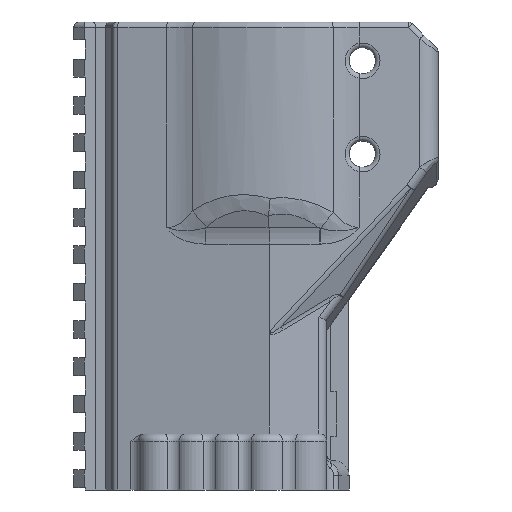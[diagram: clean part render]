
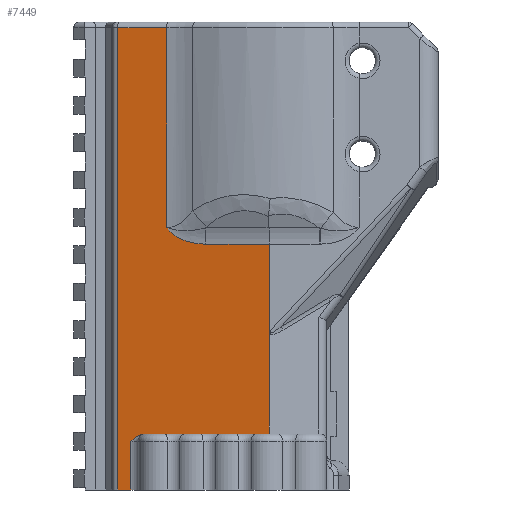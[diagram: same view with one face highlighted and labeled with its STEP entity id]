
A CAD part, left-side view. The second image highlights one B-rep face of the part: STEP entity #7449.
In plain terms, the highlighted planar face has unit normal (-0.979, 0.206, 0).
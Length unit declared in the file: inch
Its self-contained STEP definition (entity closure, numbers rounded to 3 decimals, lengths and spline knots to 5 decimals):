
#97=B_SPLINE_CURVE_WITH_KNOTS('',3,(#11676,#11677,#11678,#11679,#11680,
#11681,#11682,#11683,#11684,#11685),.UNSPECIFIED.,.F.,.F.,(4,2,2,2,4),(0.,
0.1281,0.2562,0.33578,0.41537),
 .UNSPECIFIED.);
#139=B_SPLINE_CURVE_WITH_KNOTS('',3,(#13659,#13660,#13661,#13662,#13663,
#13664,#13665,#13666,#13667,#13668,#13669,#13670),.UNSPECIFIED.,.F.,.F.,
(4,2,1,1,1,1,1,1,4),(-1.20029,-1.19791,-0.95833,
-0.83854,-0.71875,-0.59896,-0.47916,
-0.23958,0.),.UNSPECIFIED.);
#303=PLANE('',#8259);
#616=FACE_OUTER_BOUND('',#1063,.T.);
#1063=EDGE_LOOP('',(#6061,#6062,#6063,#6064,#6065,#6066,#6067,#6068,#6069,
#6070,#6071));
#1374=LINE('',#10904,#1981);
#1447=LINE('',#11693,#2054);
#1635=LINE('',#12760,#2242);
#1694=LINE('',#13674,#2301);
#1699=LINE('',#13939,#2306);
#1700=LINE('',#13941,#2307);
#1701=LINE('',#13942,#2308);
#1702=LINE('',#13943,#2309);
#1703=LINE('',#13944,#2310);
#1981=VECTOR('',#8602,0.3937);
#2054=VECTOR('',#9099,0.3937);
#2242=VECTOR('',#9643,0.3937);
#2301=VECTOR('',#9954,0.3937);
#2306=VECTOR('',#10011,0.3937);
#2307=VECTOR('',#10012,0.3937);
#2308=VECTOR('',#10013,0.3937);
#2309=VECTOR('',#10014,0.3937);
#2310=VECTOR('',#10015,0.3937);
#2996=VERTEX_POINT('',#10901);
#2997=VERTEX_POINT('',#10903);
#3186=VERTEX_POINT('',#11674);
#3187=VERTEX_POINT('',#11675);
#3189=VERTEX_POINT('',#11691);
#3456=VERTEX_POINT('',#12757);
#3457=VERTEX_POINT('',#12759);
#3545=VERTEX_POINT('',#13643);
#3547=VERTEX_POINT('',#13646);
#3562=VERTEX_POINT('',#13938);
#3563=VERTEX_POINT('',#13940);
#3711=EDGE_CURVE('',#2997,#2996,#1374,.T.);
#3956=EDGE_CURVE('',#3186,#3187,#97,.F.);
#3961=EDGE_CURVE('',#3186,#3189,#1447,.T.);
#4296=EDGE_CURVE('',#3457,#3456,#1635,.T.);
#4451=EDGE_CURVE('',#3547,#3545,#139,.T.);
#4453=EDGE_CURVE('',#3545,#3456,#1694,.T.);
#4482=EDGE_CURVE('',#3562,#3547,#1699,.T.);
#4483=EDGE_CURVE('',#3563,#3562,#1700,.T.);
#4484=EDGE_CURVE('',#2997,#3563,#1701,.T.);
#4485=EDGE_CURVE('',#3187,#2996,#1702,.T.);
#4486=EDGE_CURVE('',#3189,#3457,#1703,.T.);
#6061=ORIENTED_EDGE('',*,*,#4451,.F.);
#6062=ORIENTED_EDGE('',*,*,#4482,.F.);
#6063=ORIENTED_EDGE('',*,*,#4483,.F.);
#6064=ORIENTED_EDGE('',*,*,#4484,.F.);
#6065=ORIENTED_EDGE('',*,*,#3711,.T.);
#6066=ORIENTED_EDGE('',*,*,#4485,.F.);
#6067=ORIENTED_EDGE('',*,*,#3956,.F.);
#6068=ORIENTED_EDGE('',*,*,#3961,.T.);
#6069=ORIENTED_EDGE('',*,*,#4486,.T.);
#6070=ORIENTED_EDGE('',*,*,#4296,.T.);
#6071=ORIENTED_EDGE('',*,*,#4453,.F.);
#7449=ADVANCED_FACE('',(#616),#303,.T.);
#8259=AXIS2_PLACEMENT_3D('',#13937,#10009,#10010);
#8602=DIRECTION('',(-0.206,-0.979,0.));
#9099=DIRECTION('',(-0.206,-0.979,0.));
#9643=DIRECTION('',(0.,0.,1.));
#9954=DIRECTION('',(-0.206,-0.979,0.));
#10009=DIRECTION('center_axis',(-0.979,0.206,0.));
#10010=DIRECTION('ref_axis',(-0.206,-0.979,0.));
#10011=DIRECTION('',(0.,0.,-1.));
#10012=DIRECTION('',(-0.206,-0.979,0.));
#10013=DIRECTION('',(0.,0.,1.));
#10014=DIRECTION('',(0.,0.,-1.));
#10015=DIRECTION('',(0.,0.,1.));
#10901=CARTESIAN_POINT('',(-0.76358,0.46364,5.49557));
#10903=CARTESIAN_POINT('',(-0.73495,0.59981,5.49557));
#10904=CARTESIAN_POINT('',(-0.88188,-0.09914,5.49557));
#11674=CARTESIAN_POINT('',(-0.79501,0.31412,6.08612));
#11675=CARTESIAN_POINT('',(-0.76358,0.46364,6.01112));
#11676=CARTESIAN_POINT('Ctrl Pts',(-0.76358,0.46364,
6.01112));
#11677=CARTESIAN_POINT('Ctrl Pts',(-0.76628,0.45077,
6.0216));
#11678=CARTESIAN_POINT('Ctrl Pts',(-0.76925,0.43663,
6.03315));
#11679=CARTESIAN_POINT('Ctrl Pts',(-0.77545,0.40717,
6.05432));
#11680=CARTESIAN_POINT('Ctrl Pts',(-0.77868,0.39178,
6.06384));
#11681=CARTESIAN_POINT('Ctrl Pts',(-0.78378,0.36752,
6.07516));
#11682=CARTESIAN_POINT('Ctrl Pts',(-0.78599,0.357,
6.07918));
#11683=CARTESIAN_POINT('Ctrl Pts',(-0.79053,0.33542,
6.08467));
#11684=CARTESIAN_POINT('Ctrl Pts',(-0.79286,0.32435,
6.08612));
#11685=CARTESIAN_POINT('Ctrl Pts',(-0.79501,0.31412,
6.08612));
#11691=CARTESIAN_POINT('',(-1.07106,-0.99901,6.08612));
#11693=CARTESIAN_POINT('',(-0.8733,-0.05833,6.08612));
#12757=CARTESIAN_POINT('',(-1.07106,-0.99901,8.08939));
#12759=CARTESIAN_POINT('',(-1.07106,-0.99901,7.14465));
#12760=CARTESIAN_POINT('',(-1.07106,-0.99901,-2.40157));
#13643=CARTESIAN_POINT('',(-0.93019,-0.3289,8.08939));
#13646=CARTESIAN_POINT('',(-0.84356,0.08314,8.26572));
#13659=CARTESIAN_POINT('Ctrl Pts',(-0.84356,0.08314,
8.26572));
#13660=CARTESIAN_POINT('Ctrl Pts',(-0.8436,0.08297,
8.26546));
#13661=CARTESIAN_POINT('Ctrl Pts',(-0.84364,0.08279,
8.26521));
#13662=CARTESIAN_POINT('Ctrl Pts',(-0.84743,0.06476,
8.23931));
#13663=CARTESIAN_POINT('Ctrl Pts',(-0.85428,0.03218,
8.20509));
#13664=CARTESIAN_POINT('Ctrl Pts',(-0.86493,-0.01848,
8.16894));
#13665=CARTESIAN_POINT('Ctrl Pts',(-0.87346,-0.05908,
8.14624));
#13666=CARTESIAN_POINT('Ctrl Pts',(-0.88242,-0.1017,
8.12772));
#13667=CARTESIAN_POINT('Ctrl Pts',(-0.8948,-0.16056,
8.10823));
#13668=CARTESIAN_POINT('Ctrl Pts',(-0.91071,-0.23627,
8.09308));
#13669=CARTESIAN_POINT('Ctrl Pts',(-0.92372,-0.29814,
8.08939));
#13670=CARTESIAN_POINT('Ctrl Pts',(-0.93019,-0.3289,
8.08939));
#13674=CARTESIAN_POINT('',(-0.82801,0.15714,8.08939));
#13937=CARTESIAN_POINT('Origin',(-0.75194,0.51901,-2.40157));
#13938=CARTESIAN_POINT('',(-0.84356,0.08314,10.37402));
#13939=CARTESIAN_POINT('',(-0.84356,0.08314,10.43307));
#13940=CARTESIAN_POINT('',(-0.73495,0.59981,10.37402));
#13941=CARTESIAN_POINT('',(-0.88895,-0.13277,10.37402));
#13942=CARTESIAN_POINT('',(-0.73495,0.59981,-2.40157));
#13943=CARTESIAN_POINT('',(-0.76358,0.46364,5.49557));
#13944=CARTESIAN_POINT('',(-1.07106,-0.99901,-2.40157));
